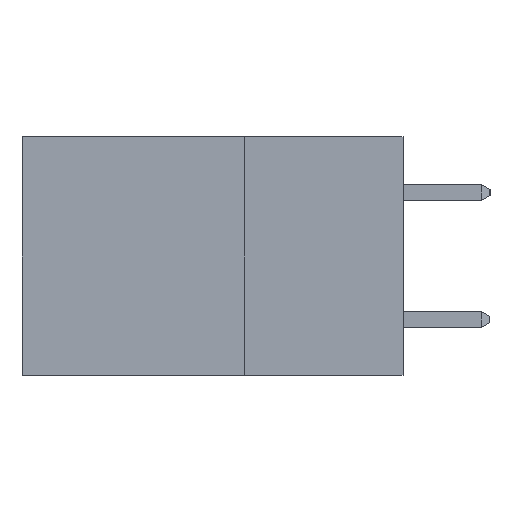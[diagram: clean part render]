
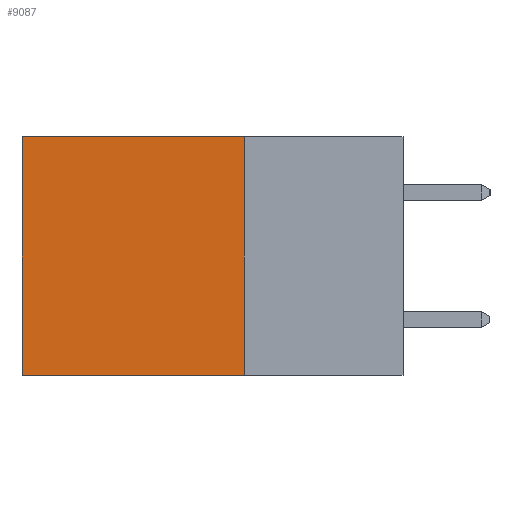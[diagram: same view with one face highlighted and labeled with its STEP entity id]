
A CAD part, left-side view. The second image highlights one B-rep face of the part: STEP entity #9087.
In plain terms, the highlighted planar face has unit normal (-1, 0, 0).
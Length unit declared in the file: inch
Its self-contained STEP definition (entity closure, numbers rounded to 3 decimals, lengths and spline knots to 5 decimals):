
#356 = ORIENTED_EDGE ( 'NONE', *, *, #1071, .T. ) ;
#1071 = EDGE_CURVE ( 'NONE', #11771, #5355, #12317, .T. ) ;
#1555 = LINE ( 'NONE', #5755, #3237 ) ;
#1568 = DIRECTION ( 'NONE',  ( 0., 1., 0. ) ) ;
#1712 = CARTESIAN_POINT ( 'NONE',  ( 0.2875, 0.6, -0.375 ) ) ;
#2019 = ORIENTED_EDGE ( 'NONE', *, *, #2670, .F. ) ;
#2670 = EDGE_CURVE ( 'NONE', #3499, #3588, #1555, .T. ) ;
#2833 = ORIENTED_EDGE ( 'NONE', *, *, #5725, .F. ) ;
#3075 = CARTESIAN_POINT ( 'NONE',  ( 0.2875, 0.25, 0. ) ) ;
#3237 = VECTOR ( 'NONE', #7911, 39.37008 ) ;
#3499 = VERTEX_POINT ( 'NONE', #9634 ) ;
#3588 = VERTEX_POINT ( 'NONE', #8925 ) ;
#4273 = EDGE_CURVE ( 'NONE', #3499, #11771, #12585, .T. ) ;
#4403 = ORIENTED_EDGE ( 'NONE', *, *, #4273, .T. ) ;
#5355 = VERTEX_POINT ( 'NONE', #7450 ) ;
#5725 = EDGE_CURVE ( 'NONE', #3588, #5355, #12118, .T. ) ;
#5755 = CARTESIAN_POINT ( 'NONE',  ( 0.2875, 0.25, -0.375 ) ) ;
#5999 = DIRECTION ( 'NONE',  ( 1., 0., 0. ) ) ;
#7450 = CARTESIAN_POINT ( 'NONE',  ( 0.2875, 0.6, -0.375 ) ) ;
#7850 = AXIS2_PLACEMENT_3D ( 'NONE', #8007, #5999, #8084 ) ;
#7911 = DIRECTION ( 'NONE',  ( 0., 0., -1. ) ) ;
#8007 = CARTESIAN_POINT ( 'NONE',  ( 0.2875, 0.25, -0.375 ) ) ;
#8084 = DIRECTION ( 'NONE',  ( 0., 0., -1. ) ) ;
#8167 = CARTESIAN_POINT ( 'NONE',  ( 0.2875, 0.6, 0. ) ) ;
#8218 = VECTOR ( 'NONE', #1568, 39.37008 ) ;
#8533 = DIRECTION ( 'NONE',  ( 0., 1., 0. ) ) ;
#8925 = CARTESIAN_POINT ( 'NONE',  ( 0.2875, 0.25, -0.375 ) ) ;
#9087 = ADVANCED_FACE ( 'NONE', ( #11295 ), #9207, .F. ) ;
#9105 = DIRECTION ( 'NONE',  ( 0., 0., -1. ) ) ;
#9207 = PLANE ( 'NONE',  #7850 ) ;
#9634 = CARTESIAN_POINT ( 'NONE',  ( 0.2875, 0.25, 0. ) ) ;
#11199 = CARTESIAN_POINT ( 'NONE',  ( 0.2875, 0.25, -0.375 ) ) ;
#11295 = FACE_OUTER_BOUND ( 'NONE', #11974, .T. ) ;
#11771 = VERTEX_POINT ( 'NONE', #8167 ) ;
#11974 = EDGE_LOOP ( 'NONE', ( #356, #2833, #2019, #4403 ) ) ;
#11985 = VECTOR ( 'NONE', #9105, 39.37008 ) ;
#12118 = LINE ( 'NONE', #11199, #8218 ) ;
#12317 = LINE ( 'NONE', #1712, #11985 ) ;
#12585 = LINE ( 'NONE', #3075, #13656 ) ;
#13656 = VECTOR ( 'NONE', #8533, 39.37008 ) ;
